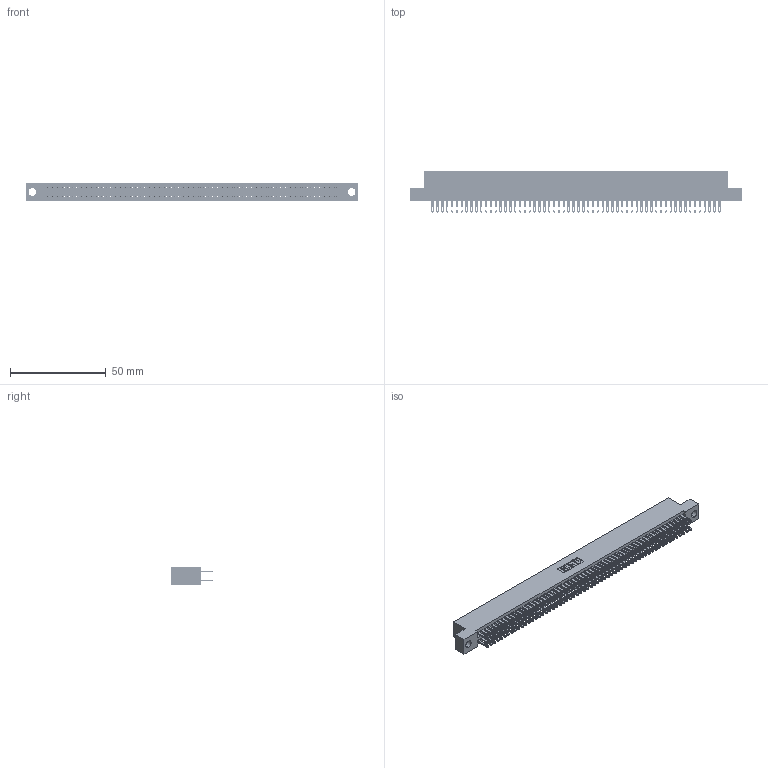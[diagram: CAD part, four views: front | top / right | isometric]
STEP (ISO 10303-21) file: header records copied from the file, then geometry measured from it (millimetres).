
FILE_DESCRIPTION (( 'STEP AP203' ), '1' );
FILE_NAME ('345-120-500-204.STEP', '2021-05-25T16:40:07', ( '' ), ( '' ), 'SwSTEP 2.0', 'SolidWorks 2020', '' );
FILE_SCHEMA (( 'CONFIG_CONTROL_DESIGN' ));
Length unit declared in the file: inch
Products named in the file (3): 345-292-001_345-293-100; 345 Part_Flush Mounting Lugs - 0.156 Dia-TI; 345-120-500-204
Assembly tree (121 placements, depth 2):
  345-120-500-204
    345 Part_Flush Mounting Lugs - 0.156 Dia-TI
    345-292-001_345-293-100  x120
Bounding box: 173.61 x 21.51 x 9.4 mm (x, y, z)
Volume: 17292.4 mm3; surface area: 26985.2 mm2
Topology: 121 solids, 121 shells, 5660 faces, 17297 edges, 11530 vertices
Faces by surface type: plane 3334, cylinder 2326
Entity records: 45003 total; most frequent: CARTESIAN_POINT 7530, ORIENTED_EDGE 7462, DIRECTION 6619, EDGE_CURVE 3731, VECTOR 3355, LINE 3355, VERTEX_POINT 2486, AXIS2_PLACEMENT_3D 1632
